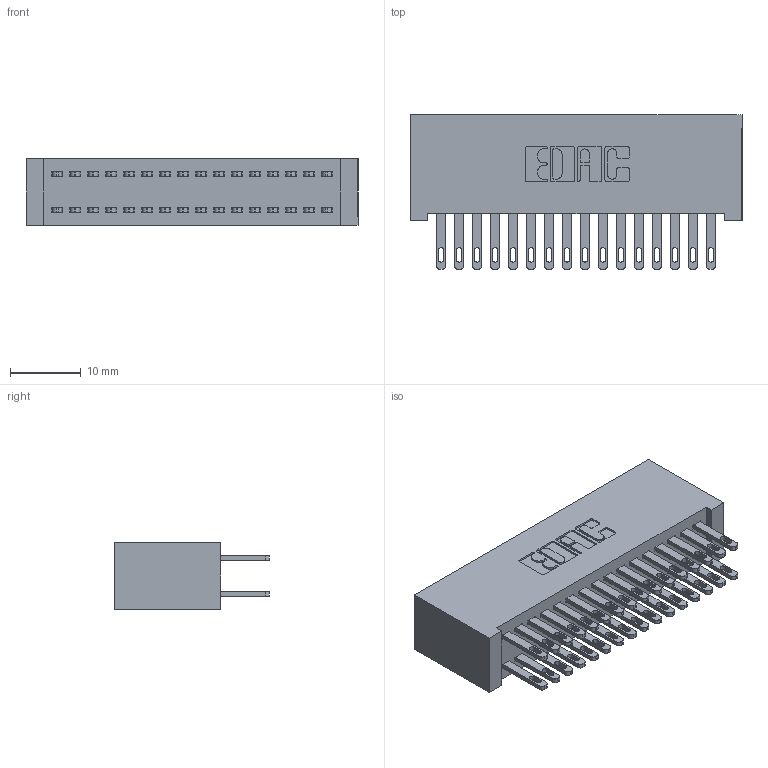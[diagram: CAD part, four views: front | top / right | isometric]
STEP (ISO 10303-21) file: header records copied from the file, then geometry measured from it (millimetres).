
FILE_DESCRIPTION (( 'STEP AP203' ), '1' );
FILE_NAME ('892-032-500-201.STEP', '2020-09-21T15:23:55', ( '' ), ( '' ), 'SwSTEP 2.0', 'SolidWorks 2020', '' );
FILE_SCHEMA (( 'CONFIG_CONTROL_DESIGN' ));
Length unit declared in the file: inch
Products named in the file (3): 842 Part_Lugless; 345-292-001_345-293-100; 892-032-500-201
Assembly tree (33 placements, depth 2):
  892-032-500-201
    842 Part_Lugless
    345-292-001_345-293-100  x32
Bounding box: 46.89 x 21.85 x 9.4 mm (x, y, z)
Volume: 4627.1 mm3; surface area: 7643.8 mm2
Topology: 33 solids, 33 shells, 1638 faces, 4979 edges, 3318 vertices
Faces by surface type: plane 1022, cylinder 616
Entity records: 13177 total; most frequent: CARTESIAN_POINT 2210, ORIENTED_EDGE 2146, DIRECTION 1929, EDGE_CURVE 1073, LINE 949, VECTOR 949, VERTEX_POINT 714, AXIS2_PLACEMENT_3D 490
